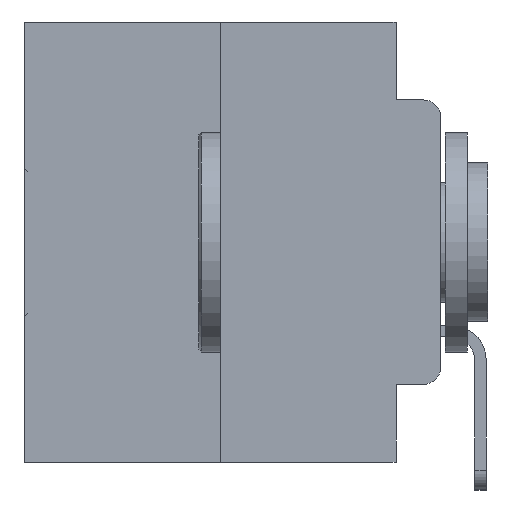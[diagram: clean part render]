
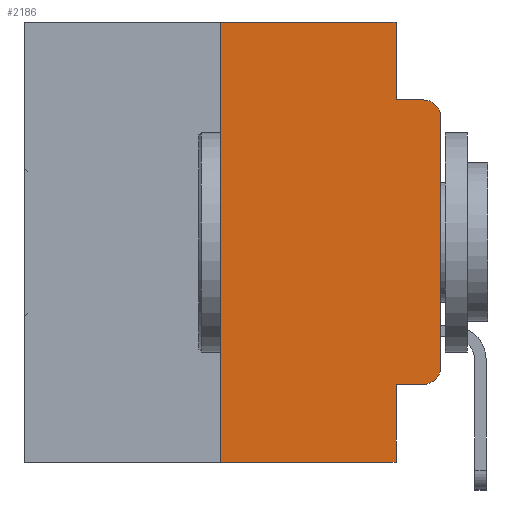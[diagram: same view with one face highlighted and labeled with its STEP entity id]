
A CAD part, left-side view. The second image highlights one B-rep face of the part: STEP entity #2186.
In plain terms, the highlighted planar face has unit normal (-1, 0, 0).
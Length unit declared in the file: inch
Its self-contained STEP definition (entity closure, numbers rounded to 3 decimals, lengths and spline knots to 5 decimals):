
#835 = VECTOR ( 'NONE', #26624, 39.37008 ) ;
#1720 = VERTEX_POINT ( 'NONE', #14356 ) ;
#2186 = ADVANCED_FACE ( 'NONE', ( #12837 ), #20272, .F. ) ;
#2498 = EDGE_CURVE ( 'NONE', #10266, #3328, #7890, .T. ) ;
#2563 = VECTOR ( 'NONE', #23964, 39.37008 ) ;
#2883 = VECTOR ( 'NONE', #19795, 39.37008 ) ;
#3326 = VERTEX_POINT ( 'NONE', #16891 ) ;
#3328 = VERTEX_POINT ( 'NONE', #30537 ) ;
#3621 = CIRCLE ( 'NONE', #8907, 0.02 ) ;
#4450 = DIRECTION ( 'NONE',  ( -1., 0., 0. ) ) ;
#5189 = ORIENTED_EDGE ( 'NONE', *, *, #7305, .F. ) ;
#5261 = ORIENTED_EDGE ( 'NONE', *, *, #11744, .F. ) ;
#5694 = CARTESIAN_POINT ( 'NONE',  ( 0., 0.02, -0.1085 ) ) ;
#6472 = VECTOR ( 'NONE', #15934, 39.37008 ) ;
#6947 = EDGE_LOOP ( 'NONE', ( #11628, #24608, #5189, #8040, #11717, #22358, #28777, #5261, #12204, #20564 ) ) ;
#7215 = LINE ( 'NONE', #27400, #6472 ) ;
#7305 = EDGE_CURVE ( 'NONE', #16681, #3328, #7215, .T. ) ;
#7731 = EDGE_CURVE ( 'NONE', #1720, #10266, #28067, .T. ) ;
#7890 = CIRCLE ( 'NONE', #19700, 0.02 ) ;
#8040 = ORIENTED_EDGE ( 'NONE', *, *, #23484, .F. ) ;
#8232 = DIRECTION ( 'NONE',  ( 0., 0., -1. ) ) ;
#8728 = CARTESIAN_POINT ( 'NONE',  ( 0., 0.051, -0.0885 ) ) ;
#8886 = VERTEX_POINT ( 'NONE', #13858 ) ;
#8907 = AXIS2_PLACEMENT_3D ( 'NONE', #18929, #4450, #21220 ) ;
#8936 = DIRECTION ( 'NONE',  ( 0., -1., 0. ) ) ;
#8956 = VECTOR ( 'NONE', #29586, 39.37008 ) ;
#10266 = VERTEX_POINT ( 'NONE', #24283 ) ;
#11002 = DIRECTION ( 'NONE',  ( 1., 0., 0. ) ) ;
#11038 = LINE ( 'NONE', #12943, #28091 ) ;
#11063 = EDGE_CURVE ( 'NONE', #21723, #16929, #15774, .T. ) ;
#11086 = CARTESIAN_POINT ( 'NONE',  ( 0., 0.473, 0. ) ) ;
#11628 = ORIENTED_EDGE ( 'NONE', *, *, #7731, .T. ) ;
#11717 = ORIENTED_EDGE ( 'NONE', *, *, #21701, .F. ) ;
#11744 = EDGE_CURVE ( 'NONE', #22186, #16929, #15369, .T. ) ;
#12204 = ORIENTED_EDGE ( 'NONE', *, *, #14945, .T. ) ;
#12420 = DIRECTION ( 'NONE',  ( 0., -1., 0. ) ) ;
#12837 = FACE_OUTER_BOUND ( 'NONE', #6947, .T. ) ;
#12943 = CARTESIAN_POINT ( 'NONE',  ( 0., 0.25, 0. ) ) ;
#13858 = CARTESIAN_POINT ( 'NONE',  ( 0., 0.051, 0. ) ) ;
#14356 = CARTESIAN_POINT ( 'NONE',  ( 0., 0., -0.3915 ) ) ;
#14945 = EDGE_CURVE ( 'NONE', #22186, #3326, #23444, .T. ) ;
#15305 = LINE ( 'NONE', #11086, #8956 ) ;
#15369 = LINE ( 'NONE', #31154, #2883 ) ;
#15534 = EDGE_CURVE ( 'NONE', #21723, #16853, #11038, .T. ) ;
#15774 = LINE ( 'NONE', #23959, #27295 ) ;
#15934 = DIRECTION ( 'NONE',  ( 0., -1., 0. ) ) ;
#16681 = VERTEX_POINT ( 'NONE', #8728 ) ;
#16853 = VERTEX_POINT ( 'NONE', #25611 ) ;
#16891 = CARTESIAN_POINT ( 'NONE',  ( 0., 0.02, -0.4115 ) ) ;
#16929 = VERTEX_POINT ( 'NONE', #28163 ) ;
#17259 = CARTESIAN_POINT ( 'NONE',  ( 0., 0.051, -0.4115 ) ) ;
#17345 = VECTOR ( 'NONE', #8936, 39.37008 ) ;
#18169 = CARTESIAN_POINT ( 'NONE',  ( 0., 0.25, -0.5 ) ) ;
#18929 = CARTESIAN_POINT ( 'NONE',  ( 0., 0.02, -0.3915 ) ) ;
#19301 = AXIS2_PLACEMENT_3D ( 'NONE', #24908, #11002, #27217 ) ;
#19700 = AXIS2_PLACEMENT_3D ( 'NONE', #5694, #22255, #8232 ) ;
#19795 = DIRECTION ( 'NONE',  ( 0., 0., -1. ) ) ;
#20272 = PLANE ( 'NONE',  #19301 ) ;
#20525 = LINE ( 'NONE', #28948, #835 ) ;
#20564 = ORIENTED_EDGE ( 'NONE', *, *, #22650, .T. ) ;
#21220 = DIRECTION ( 'NONE',  ( 0., 0., -1. ) ) ;
#21638 = CARTESIAN_POINT ( 'NONE',  ( 0., 0., 0. ) ) ;
#21701 = EDGE_CURVE ( 'NONE', #16853, #8886, #15305, .T. ) ;
#21723 = VERTEX_POINT ( 'NONE', #18169 ) ;
#22186 = VERTEX_POINT ( 'NONE', #17259 ) ;
#22255 = DIRECTION ( 'NONE',  ( -1., 0., 0. ) ) ;
#22358 = ORIENTED_EDGE ( 'NONE', *, *, #15534, .F. ) ;
#22650 = EDGE_CURVE ( 'NONE', #3326, #1720, #3621, .T. ) ;
#23444 = LINE ( 'NONE', #29738, #17345 ) ;
#23484 = EDGE_CURVE ( 'NONE', #8886, #16681, #20525, .T. ) ;
#23959 = CARTESIAN_POINT ( 'NONE',  ( 0., 0.473, -0.5 ) ) ;
#23964 = DIRECTION ( 'NONE',  ( 0., 0., 1. ) ) ;
#24283 = CARTESIAN_POINT ( 'NONE',  ( 0., 0., -0.1085 ) ) ;
#24608 = ORIENTED_EDGE ( 'NONE', *, *, #2498, .T. ) ;
#24908 = CARTESIAN_POINT ( 'NONE',  ( 0., 0.473, 0. ) ) ;
#25611 = CARTESIAN_POINT ( 'NONE',  ( 0., 0.25, 0. ) ) ;
#26624 = DIRECTION ( 'NONE',  ( 0., 0., -1. ) ) ;
#26739 = DIRECTION ( 'NONE',  ( 0., 0., 1. ) ) ;
#27217 = DIRECTION ( 'NONE',  ( 0., 0., -1. ) ) ;
#27295 = VECTOR ( 'NONE', #12420, 39.37008 ) ;
#27400 = CARTESIAN_POINT ( 'NONE',  ( 0., 0.051, -0.0885 ) ) ;
#28067 = LINE ( 'NONE', #21638, #2563 ) ;
#28091 = VECTOR ( 'NONE', #26739, 39.37008 ) ;
#28163 = CARTESIAN_POINT ( 'NONE',  ( 0., 0.051, -0.5 ) ) ;
#28777 = ORIENTED_EDGE ( 'NONE', *, *, #11063, .T. ) ;
#28948 = CARTESIAN_POINT ( 'NONE',  ( 0., 0.051, 0. ) ) ;
#29586 = DIRECTION ( 'NONE',  ( 0., -1., 0. ) ) ;
#29738 = CARTESIAN_POINT ( 'NONE',  ( 0., 0.051, -0.4115 ) ) ;
#30537 = CARTESIAN_POINT ( 'NONE',  ( 0., 0.02, -0.0885 ) ) ;
#31154 = CARTESIAN_POINT ( 'NONE',  ( 0., 0.051, 0. ) ) ;
